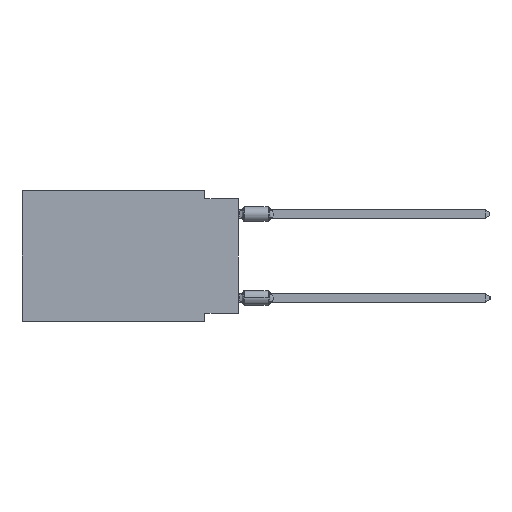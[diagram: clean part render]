
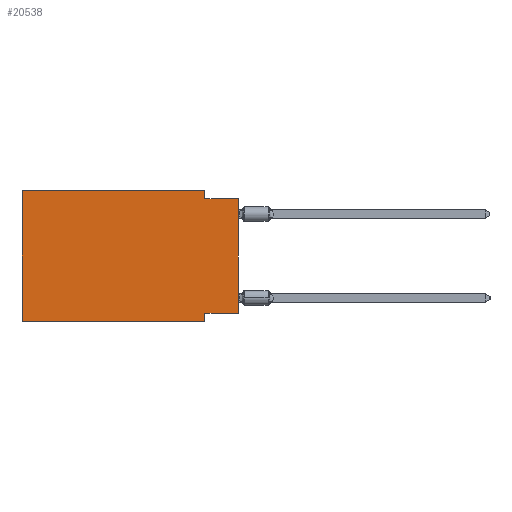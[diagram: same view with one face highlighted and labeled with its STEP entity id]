
A CAD part, left-side view. The second image highlights one B-rep face of the part: STEP entity #20538.
In plain terms, the highlighted planar face has unit normal (-1, 0, 0).
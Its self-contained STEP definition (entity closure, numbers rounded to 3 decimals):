
#901 = ORIENTED_EDGE ( 'NONE', *, *, #9460, .F. ) ;
#1505 = EDGE_CURVE ( 'NONE', #31460, #33280, #13077, .T. ) ;
#2288 = ORIENTED_EDGE ( 'NONE', *, *, #23794, .F. ) ;
#2499 = VECTOR ( 'NONE', #22581, 1000. ) ;
#2526 = CARTESIAN_POINT ( 'NONE',  ( 0., 0., -9.271 ) ) ;
#2545 = CARTESIAN_POINT ( 'NONE',  ( 0., 2.54, -9.906 ) ) ;
#2781 = CARTESIAN_POINT ( 'NONE',  ( 0., 16.383, -9.906 ) ) ;
#2841 = FACE_OUTER_BOUND ( 'NONE', #23996, .T. ) ;
#3519 = EDGE_CURVE ( 'NONE', #9249, #5110, #22374, .T. ) ;
#3738 = PLANE ( 'NONE',  #14761 ) ;
#4229 = VECTOR ( 'NONE', #16482, 1000. ) ;
#4976 = DIRECTION ( 'NONE',  ( 0., 0., 1. ) ) ;
#5110 = VERTEX_POINT ( 'NONE', #22846 ) ;
#5307 = CARTESIAN_POINT ( 'NONE',  ( 0., 2.54, -0.635 ) ) ;
#5967 = DIRECTION ( 'NONE',  ( 0., 0., -1. ) ) ;
#6443 = VECTOR ( 'NONE', #21992, 1000. ) ;
#6491 = ORIENTED_EDGE ( 'NONE', *, *, #44919, .F. ) ;
#8037 = CARTESIAN_POINT ( 'NONE',  ( 0., 16.383, 0. ) ) ;
#9249 = VERTEX_POINT ( 'NONE', #43478 ) ;
#9460 = EDGE_CURVE ( 'NONE', #40141, #31460, #19913, .T. ) ;
#9688 = VECTOR ( 'NONE', #30887, 1000. ) ;
#10512 = DIRECTION ( 'NONE',  ( 0., 1., 0. ) ) ;
#10577 = VECTOR ( 'NONE', #22543, 1000. ) ;
#12152 = CARTESIAN_POINT ( 'NONE',  ( 0., 2.54, 0. ) ) ;
#12494 = EDGE_CURVE ( 'NONE', #32989, #13612, #25302, .T. ) ;
#13077 = LINE ( 'NONE', #2545, #36415 ) ;
#13612 = VERTEX_POINT ( 'NONE', #37955 ) ;
#13835 = ORIENTED_EDGE ( 'NONE', *, *, #28854, .T. ) ;
#14761 = AXIS2_PLACEMENT_3D ( 'NONE', #38504, #27773, #37818 ) ;
#15135 = VECTOR ( 'NONE', #10512, 1000. ) ;
#15510 = CARTESIAN_POINT ( 'NONE',  ( 0., 16.383, 0. ) ) ;
#16482 = DIRECTION ( 'NONE',  ( 0., 0., -1. ) ) ;
#16910 = CARTESIAN_POINT ( 'NONE',  ( 0., 0., -9.271 ) ) ;
#16957 = LINE ( 'NONE', #2781, #9688 ) ;
#17760 = ORIENTED_EDGE ( 'NONE', *, *, #3519, .F. ) ;
#17812 = CARTESIAN_POINT ( 'NONE',  ( 0., 2.54, 0. ) ) ;
#19142 = CARTESIAN_POINT ( 'NONE',  ( 0., 0., 0. ) ) ;
#19913 = LINE ( 'NONE', #2526, #15135 ) ;
#20538 = ADVANCED_FACE ( 'NONE', ( #2841 ), #3738, .F. ) ;
#20848 = ORIENTED_EDGE ( 'NONE', *, *, #1505, .F. ) ;
#21992 = DIRECTION ( 'NONE',  ( 0., -1., 0. ) ) ;
#22374 = LINE ( 'NONE', #15510, #41578 ) ;
#22543 = DIRECTION ( 'NONE',  ( 0., -1., 0. ) ) ;
#22581 = DIRECTION ( 'NONE',  ( 0., 0., 1. ) ) ;
#22846 = CARTESIAN_POINT ( 'NONE',  ( 0., 16.383, 0. ) ) ;
#23221 = CARTESIAN_POINT ( 'NONE',  ( 0., 2.54, -9.271 ) ) ;
#23794 = EDGE_CURVE ( 'NONE', #29445, #32989, #37272, .T. ) ;
#23996 = EDGE_LOOP ( 'NONE', ( #24822, #32243, #2288, #6491, #17760, #13835, #20848, #901 ) ) ;
#24822 = ORIENTED_EDGE ( 'NONE', *, *, #37852, .T. ) ;
#25302 = LINE ( 'NONE', #29184, #10577 ) ;
#27773 = DIRECTION ( 'NONE',  ( 1., 0., 0. ) ) ;
#28854 = EDGE_CURVE ( 'NONE', #9249, #33280, #16957, .T. ) ;
#29184 = CARTESIAN_POINT ( 'NONE',  ( 0., 0., -0.635 ) ) ;
#29445 = VERTEX_POINT ( 'NONE', #17812 ) ;
#30887 = DIRECTION ( 'NONE',  ( 0., -1., 0. ) ) ;
#31460 = VERTEX_POINT ( 'NONE', #23221 ) ;
#32047 = LINE ( 'NONE', #8037, #6443 ) ;
#32243 = ORIENTED_EDGE ( 'NONE', *, *, #12494, .F. ) ;
#32989 = VERTEX_POINT ( 'NONE', #5307 ) ;
#33280 = VERTEX_POINT ( 'NONE', #36140 ) ;
#36140 = CARTESIAN_POINT ( 'NONE',  ( 0., 2.54, -9.906 ) ) ;
#36415 = VECTOR ( 'NONE', #5967, 1000. ) ;
#37272 = LINE ( 'NONE', #12152, #4229 ) ;
#37818 = DIRECTION ( 'NONE',  ( 0., 0., -1. ) ) ;
#37852 = EDGE_CURVE ( 'NONE', #40141, #13612, #39953, .T. ) ;
#37955 = CARTESIAN_POINT ( 'NONE',  ( 0., 0., -0.635 ) ) ;
#38504 = CARTESIAN_POINT ( 'NONE',  ( 0., 16.383, 0. ) ) ;
#39953 = LINE ( 'NONE', #19142, #2499 ) ;
#40141 = VERTEX_POINT ( 'NONE', #16910 ) ;
#41578 = VECTOR ( 'NONE', #4976, 1000. ) ;
#43478 = CARTESIAN_POINT ( 'NONE',  ( 0., 16.383, -9.906 ) ) ;
#44919 = EDGE_CURVE ( 'NONE', #5110, #29445, #32047, .T. ) ;
